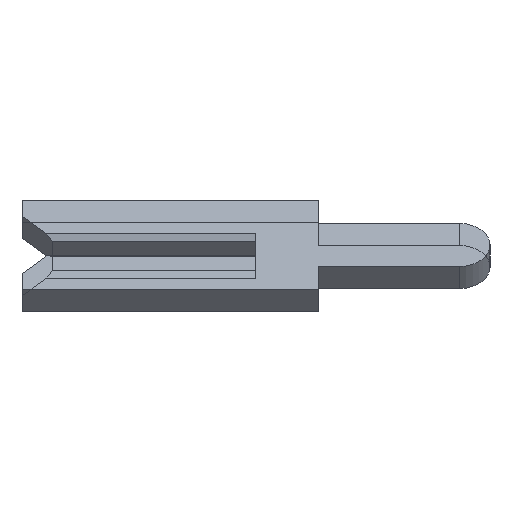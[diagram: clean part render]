
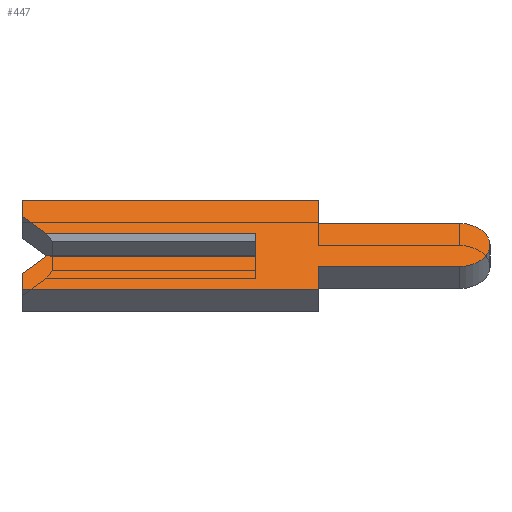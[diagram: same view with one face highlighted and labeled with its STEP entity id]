
A CAD part, left-side view. The second image highlights one B-rep face of the part: STEP entity #447.
In plain terms, the highlighted face is planar.
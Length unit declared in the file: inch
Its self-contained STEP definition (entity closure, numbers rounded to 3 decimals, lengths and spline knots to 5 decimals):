
#7 = VECTOR ( 'NONE', #614, 39.37008 ) ;
#31 = DIRECTION ( 'NONE',  ( 1., 0., 0. ) ) ;
#44 = DIRECTION ( 'NONE',  ( 0., 0.707, 0.707 ) ) ;
#71 = DIRECTION ( 'NONE',  ( 0., 1., 0. ) ) ;
#100 = VECTOR ( 'NONE', #44, 39.37008 ) ;
#106 = DIRECTION ( 'NONE',  ( 0., -1., 0. ) ) ;
#115 = DIRECTION ( 'NONE',  ( 0., 0., -1. ) ) ;
#129 = LINE ( 'NONE', #2208, #100 ) ;
#208 = LINE ( 'NONE', #2320, #2026 ) ;
#210 = DIRECTION ( 'NONE',  ( 0., -1., 0. ) ) ;
#218 = LINE ( 'NONE', #1749, #1733 ) ;
#230 = CARTESIAN_POINT ( 'NONE',  ( -0.01, -0.1305, 0.0195 ) ) ;
#231 = EDGE_CURVE ( 'NONE', #2495, #550, #1924, .T. ) ;
#253 = LINE ( 'NONE', #529, #2547 ) ;
#287 = EDGE_CURVE ( 'NONE', #1995, #2495, #208, .T. ) ;
#304 = CARTESIAN_POINT ( 'NONE',  ( -0.01, 0., 0.0065 ) ) ;
#314 = EDGE_CURVE ( 'NONE', #2184, #531, #1026, .T. ) ;
#339 = CARTESIAN_POINT ( 'NONE',  ( -0.01, 0.134, -0.01 ) ) ;
#347 = CARTESIAN_POINT ( 'NONE',  ( -0.01, 0.15, -0.04 ) ) ;
#357 = DIRECTION ( 'NONE',  ( 0., 1., 0. ) ) ;
#388 = ORIENTED_EDGE ( 'NONE', *, *, #1616, .F. ) ;
#416 = ORIENTED_EDGE ( 'NONE', *, *, #641, .F. ) ;
#421 = AXIS2_PLACEMENT_3D ( 'NONE', #1303, #31, #1076 ) ;
#447 = ADVANCED_FACE ( 'NONE', ( #2628 ), #1491, .F. ) ;
#469 = LINE ( 'NONE', #1137, #858 ) ;
#473 = ORIENTED_EDGE ( 'NONE', *, *, #1543, .F. ) ;
#477 = DIRECTION ( 'NONE',  ( 0., -1., 0. ) ) ;
#505 = LINE ( 'NONE', #862, #1363 ) ;
#529 = CARTESIAN_POINT ( 'NONE',  ( -0.01, 0.1305, -0.0065 ) ) ;
#531 = VERTEX_POINT ( 'NONE', #640 ) ;
#545 = CARTESIAN_POINT ( 'NONE',  ( -0.01, -0.1305, -0.0195 ) ) ;
#550 = VERTEX_POINT ( 'NONE', #1711 ) ;
#586 = DIRECTION ( 'NONE',  ( 0., 0., 1. ) ) ;
#610 = ORIENTED_EDGE ( 'NONE', *, *, #1136, .F. ) ;
#614 = DIRECTION ( 'NONE',  ( 0., -1., 0. ) ) ;
#640 = CARTESIAN_POINT ( 'NONE',  ( -0.01, 0.15, -0.026 ) ) ;
#641 = EDGE_CURVE ( 'NONE', #1906, #2641, #505, .T. ) ;
#645 = ORIENTED_EDGE ( 'NONE', *, *, #287, .F. ) ;
#676 = EDGE_CURVE ( 'NONE', #2020, #1595, #469, .T. ) ;
#710 = EDGE_LOOP ( 'NONE', ( #865, #388, #2408, #1576, #778, #1618, #1452, #1245, #1017, #416, #473, #2245, #645, #610 ) ) ;
#725 = LINE ( 'NONE', #1790, #1998 ) ;
#748 = CARTESIAN_POINT ( 'NONE',  ( -0.01, -0.1305, 0. ) ) ;
#778 = ORIENTED_EDGE ( 'NONE', *, *, #314, .F. ) ;
#792 = CARTESIAN_POINT ( 'NONE',  ( -0.01, 0.15, 0.04 ) ) ;
#796 = DIRECTION ( 'NONE',  ( 0., 0., 1. ) ) ;
#807 = EDGE_CURVE ( 'NONE', #1591, #2184, #218, .T. ) ;
#853 = VECTOR ( 'NONE', #357, 39.37008 ) ;
#858 = VECTOR ( 'NONE', #477, 39.37008 ) ;
#862 = CARTESIAN_POINT ( 'NONE',  ( -0.01, -0.04, 0.0195 ) ) ;
#865 = ORIENTED_EDGE ( 'NONE', *, *, #676, .T. ) ;
#889 = VECTOR ( 'NONE', #586, 39.37008 ) ;
#938 = DIRECTION ( 'NONE',  ( 0., 0., 1. ) ) ;
#990 = CARTESIAN_POINT ( 'NONE',  ( -0.01, -0.04, 0.0195 ) ) ;
#1017 = ORIENTED_EDGE ( 'NONE', *, *, #1219, .F. ) ;
#1026 = LINE ( 'NONE', #1895, #889 ) ;
#1061 = CIRCLE ( 'NONE', #2622, 0.0195 ) ;
#1076 = DIRECTION ( 'NONE',  ( 0., 0., -1. ) ) ;
#1136 = EDGE_CURVE ( 'NONE', #2020, #1995, #129, .T. ) ;
#1137 = CARTESIAN_POINT ( 'NONE',  ( -0.01, 0.15, 0.01 ) ) ;
#1191 = VECTOR ( 'NONE', #115, 39.37008 ) ;
#1219 = EDGE_CURVE ( 'NONE', #2641, #1397, #1061, .T. ) ;
#1241 = CARTESIAN_POINT ( 'NONE',  ( -0.01, -0.04, -0.04 ) ) ;
#1245 = ORIENTED_EDGE ( 'NONE', *, *, #1759, .F. ) ;
#1276 = EDGE_CURVE ( 'NONE', #2022, #1280, #725, .T. ) ;
#1280 = VERTEX_POINT ( 'NONE', #1356 ) ;
#1303 = CARTESIAN_POINT ( 'NONE',  ( -0.01, -0.1305, 0. ) ) ;
#1356 = CARTESIAN_POINT ( 'NONE',  ( -0.01, 0., -0.01 ) ) ;
#1363 = VECTOR ( 'NONE', #210, 39.37008 ) ;
#1379 = CARTESIAN_POINT ( 'NONE',  ( -0.01, -0.04, -0.0195 ) ) ;
#1391 = DIRECTION ( 'NONE',  ( 0., -0.707, 0.707 ) ) ;
#1397 = VERTEX_POINT ( 'NONE', #545 ) ;
#1432 = CARTESIAN_POINT ( 'NONE',  ( -0.01, 0.134, 0.01 ) ) ;
#1452 = ORIENTED_EDGE ( 'NONE', *, *, #2571, .F. ) ;
#1489 = EDGE_CURVE ( 'NONE', #531, #2022, #253, .T. ) ;
#1491 = PLANE ( 'NONE',  #421 ) ;
#1543 = EDGE_CURVE ( 'NONE', #550, #1906, #1637, .T. ) ;
#1576 = ORIENTED_EDGE ( 'NONE', *, *, #1489, .F. ) ;
#1591 = VERTEX_POINT ( 'NONE', #2421 ) ;
#1595 = VERTEX_POINT ( 'NONE', #2461 ) ;
#1616 = EDGE_CURVE ( 'NONE', #1280, #1595, #2623, .T. ) ;
#1618 = ORIENTED_EDGE ( 'NONE', *, *, #807, .F. ) ;
#1637 = LINE ( 'NONE', #2015, #1191 ) ;
#1711 = CARTESIAN_POINT ( 'NONE',  ( -0.01, -0.04, 0.04 ) ) ;
#1725 = DIRECTION ( 'NONE',  ( 0., 0., -1. ) ) ;
#1733 = VECTOR ( 'NONE', #71, 39.37008 ) ;
#1749 = CARTESIAN_POINT ( 'NONE',  ( -0.01, 0.15, -0.04 ) ) ;
#1759 = EDGE_CURVE ( 'NONE', #1397, #2613, #2585, .T. ) ;
#1790 = CARTESIAN_POINT ( 'NONE',  ( -0.01, -0.1305, -0.01 ) ) ;
#1883 = CARTESIAN_POINT ( 'NONE',  ( -0.01, -0.04, -0.0195 ) ) ;
#1884 = CARTESIAN_POINT ( 'NONE',  ( -0.01, 0.15, 0.04 ) ) ;
#1895 = CARTESIAN_POINT ( 'NONE',  ( -0.01, 0.15, -0.026 ) ) ;
#1906 = VERTEX_POINT ( 'NONE', #990 ) ;
#1922 = VECTOR ( 'NONE', #1725, 39.37008 ) ;
#1924 = LINE ( 'NONE', #1884, #7 ) ;
#1993 = VECTOR ( 'NONE', #938, 39.37008 ) ;
#1995 = VERTEX_POINT ( 'NONE', #2112 ) ;
#1998 = VECTOR ( 'NONE', #106, 39.37008 ) ;
#2015 = CARTESIAN_POINT ( 'NONE',  ( -0.01, -0.04, 0.04 ) ) ;
#2020 = VERTEX_POINT ( 'NONE', #1432 ) ;
#2022 = VERTEX_POINT ( 'NONE', #339 ) ;
#2026 = VECTOR ( 'NONE', #796, 39.37008 ) ;
#2032 = LINE ( 'NONE', #1241, #1922 ) ;
#2112 = CARTESIAN_POINT ( 'NONE',  ( -0.01, 0.15, 0.026 ) ) ;
#2184 = VERTEX_POINT ( 'NONE', #347 ) ;
#2208 = CARTESIAN_POINT ( 'NONE',  ( -0.01, 0.1305, 0.0065 ) ) ;
#2219 = DIRECTION ( 'NONE',  ( 0., 0., -1. ) ) ;
#2245 = ORIENTED_EDGE ( 'NONE', *, *, #231, .F. ) ;
#2320 = CARTESIAN_POINT ( 'NONE',  ( -0.01, 0.15, 0.026 ) ) ;
#2408 = ORIENTED_EDGE ( 'NONE', *, *, #1276, .F. ) ;
#2421 = CARTESIAN_POINT ( 'NONE',  ( -0.01, -0.04, -0.04 ) ) ;
#2461 = CARTESIAN_POINT ( 'NONE',  ( -0.01, 0., 0.01 ) ) ;
#2495 = VERTEX_POINT ( 'NONE', #792 ) ;
#2547 = VECTOR ( 'NONE', #1391, 39.37008 ) ;
#2571 = EDGE_CURVE ( 'NONE', #2613, #1591, #2032, .T. ) ;
#2585 = LINE ( 'NONE', #1379, #853 ) ;
#2613 = VERTEX_POINT ( 'NONE', #1883 ) ;
#2622 = AXIS2_PLACEMENT_3D ( 'NONE', #748, #2668, #2219 ) ;
#2623 = LINE ( 'NONE', #304, #1993 ) ;
#2628 = FACE_OUTER_BOUND ( 'NONE', #710, .T. ) ;
#2641 = VERTEX_POINT ( 'NONE', #230 ) ;
#2668 = DIRECTION ( 'NONE',  ( 1., 0., 0. ) ) ;
